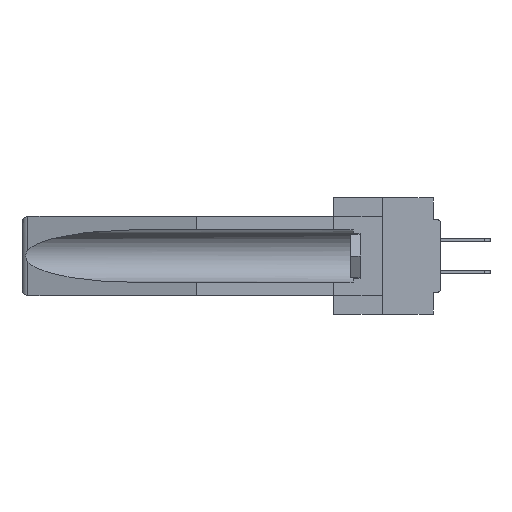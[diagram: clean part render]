
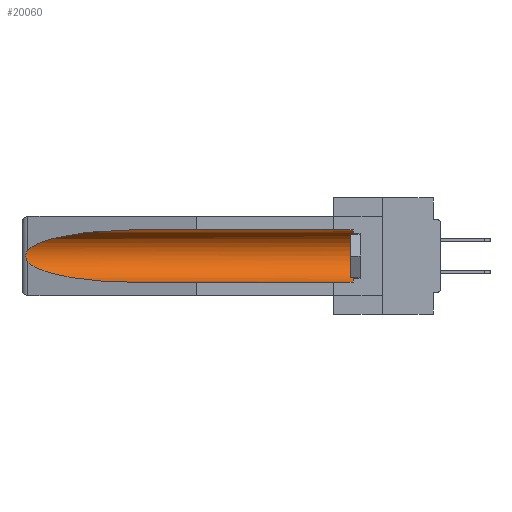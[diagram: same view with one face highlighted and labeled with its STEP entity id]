
A CAD part, left-side view. The second image highlights one B-rep face of the part: STEP entity #20060.
In plain terms, the highlighted cylindrical face has radius 2.857 mm (diameter 5.715 mm), a partial arc.
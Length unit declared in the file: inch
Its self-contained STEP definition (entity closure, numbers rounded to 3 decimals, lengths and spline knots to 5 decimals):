
#20 = CARTESIAN_POINT ( 'NONE',  ( 0.21114, 1.30732, -0.284 ) ) ;
#1206 = CARTESIAN_POINT ( 'NONE',  ( 0.26537, 1.52718, -0.14972 ) ) ;
#1424 = EDGE_CURVE ( 'NONE', #20985, #10053, #11545, .T. ) ;
#1630 = EDGE_CURVE ( 'NONE', #35084, #40783, #12190, .T. ) ;
#1663 = CARTESIAN_POINT ( 'NONE',  ( 0.25451, 1.48313, -0.09465 ) ) ;
#2729 = DIRECTION ( 'NONE',  ( 0., 1., 0. ) ) ;
#2891 = CARTESIAN_POINT ( 'NONE',  ( 0.155, 1.07973, -0.059 ) ) ;
#5031 = DIRECTION ( 'NONE',  ( 0., 1., 0. ) ) ;
#5804 = CARTESIAN_POINT ( 'NONE',  ( 0.2675, 1.53308, -0.16763 ) ) ;
#6280 = VERTEX_POINT ( 'NONE', #25999 ) ;
#8347 = VERTEX_POINT ( 'NONE', #2891 ) ;
#8759 = EDGE_CURVE ( 'NONE', #8347, #35084, #24350, .T. ) ;
#9549 = EDGE_CURVE ( 'NONE', #40783, #10053, #16324, .T. ) ;
#9585 = ORIENTED_EDGE ( 'NONE', *, *, #8759, .T. ) ;
#9876 = CARTESIAN_POINT ( 'NONE',  ( 0.26537, 1.52718, -0.19328 ) ) ;
#10053 = VERTEX_POINT ( 'NONE', #32506 ) ;
#11545 = LINE ( 'NONE', #38792, #32126 ) ;
#12190 = B_SPLINE_CURVE_WITH_KNOTS ( 'NONE', 3,
 ( #27003, #30457, #13221, #40988, #5804, #16128, #20136, #27146, #44496, #23081 ),
 .UNSPECIFIED., .F., .F.,
 ( 4, 2, 2, 2, 4 ),
 ( 0., 0.00029, 0.00058, 0.00087, 0.00117 ),
 .UNSPECIFIED. ) ;
#13221 = CARTESIAN_POINT ( 'NONE',  ( 0.26654, 1.53092, -0.15636 ) ) ;
#13611 = CARTESIAN_POINT ( 'NONE',  ( 0.155, 0.126, -0.1715 ) ) ;
#15307 = CYLINDRICAL_SURFACE ( 'NONE', #31145, 0.1125 ) ;
#16128 = CARTESIAN_POINT ( 'NONE',  ( 0.2675, 1.53308, -0.17534 ) ) ;
#16324 =( BOUNDED_CURVE ( )  B_SPLINE_CURVE ( 3, ( #39674, #37750, #20, #20393 ),
 .UNSPECIFIED., .F., .F. ) 
 B_SPLINE_CURVE_WITH_KNOTS ( ( 4, 4 ),
 ( 0.1948, 1.5708 ),
 .UNSPECIFIED. ) 
 CURVE ( )  GEOMETRIC_REPRESENTATION_ITEM ( )  RATIONAL_B_SPLINE_CURVE ( ( 1., 0.848, 0.848, 1. ) ) 
 REPRESENTATION_ITEM ( '' )  );
#16399 = FACE_OUTER_BOUND ( 'NONE', #27648, .T. ) ;
#16634 = ORIENTED_EDGE ( 'NONE', *, *, #1630, .T. ) ;
#19645 = DIRECTION ( 'NONE',  ( 0., 0., 1. ) ) ;
#20060 = ADVANCED_FACE ( 'NONE', ( #16399 ), #15307, .F. ) ;
#20136 = CARTESIAN_POINT ( 'NONE',  ( 0.2673, 1.53269, -0.17917 ) ) ;
#20393 = CARTESIAN_POINT ( 'NONE',  ( 0.155, 1.07973, -0.284 ) ) ;
#20543 = DIRECTION ( 'NONE',  ( 0., 0., 1. ) ) ;
#20985 = VERTEX_POINT ( 'NONE', #24520 ) ;
#21952 = VECTOR ( 'NONE', #5031, 39.37008 ) ;
#23081 = CARTESIAN_POINT ( 'NONE',  ( 0.26537, 1.52718, -0.19328 ) ) ;
#23207 = ORIENTED_EDGE ( 'NONE', *, *, #23933, .T. ) ;
#23933 = EDGE_CURVE ( 'NONE', #6280, #8347, #32287, .T. ) ;
#24350 =( BOUNDED_CURVE ( )  B_SPLINE_CURVE ( 3, ( #39292, #43068, #1663, #1206 ),
 .UNSPECIFIED., .F., .F. ) 
 B_SPLINE_CURVE_WITH_KNOTS ( ( 4, 4 ),
 ( 4.71239, 6.08839 ),
 .UNSPECIFIED. ) 
 CURVE ( )  GEOMETRIC_REPRESENTATION_ITEM ( )  RATIONAL_B_SPLINE_CURVE ( ( 1., 0.848, 0.848, 1. ) ) 
 REPRESENTATION_ITEM ( '' )  );
#24520 = CARTESIAN_POINT ( 'NONE',  ( 0.155, 0.126, -0.284 ) ) ;
#25999 = CARTESIAN_POINT ( 'NONE',  ( 0.155, 0.126, -0.059 ) ) ;
#27003 = CARTESIAN_POINT ( 'NONE',  ( 0.26537, 1.52718, -0.14972 ) ) ;
#27146 = CARTESIAN_POINT ( 'NONE',  ( 0.26655, 1.53094, -0.18657 ) ) ;
#27648 = EDGE_LOOP ( 'NONE', ( #9585, #16634, #31388, #28370, #41620, #23207 ) ) ;
#28370 = ORIENTED_EDGE ( 'NONE', *, *, #1424, .F. ) ;
#30457 = CARTESIAN_POINT ( 'NONE',  ( 0.26597, 1.52961, -0.15275 ) ) ;
#31145 = AXIS2_PLACEMENT_3D ( 'NONE', #34068, #2729, #19645 ) ;
#31388 = ORIENTED_EDGE ( 'NONE', *, *, #9549, .T. ) ;
#32126 = VECTOR ( 'NONE', #42091, 39.37008 ) ;
#32287 = LINE ( 'NONE', #35805, #21952 ) ;
#32506 = CARTESIAN_POINT ( 'NONE',  ( 0.155, 1.07973, -0.284 ) ) ;
#32802 = CARTESIAN_POINT ( 'NONE',  ( 0.26537, 1.52718, -0.14972 ) ) ;
#34068 = CARTESIAN_POINT ( 'NONE',  ( 0.155, -0.30754, -0.1715 ) ) ;
#35084 = VERTEX_POINT ( 'NONE', #32802 ) ;
#35805 = CARTESIAN_POINT ( 'NONE',  ( 0.155, -0.30754, -0.059 ) ) ;
#37076 = CIRCLE ( 'NONE', #39961, 0.1125 ) ;
#37750 = CARTESIAN_POINT ( 'NONE',  ( 0.25451, 1.48313, -0.24835 ) ) ;
#38792 = CARTESIAN_POINT ( 'NONE',  ( 0.155, -0.30754, -0.284 ) ) ;
#39292 = CARTESIAN_POINT ( 'NONE',  ( 0.155, 1.07973, -0.059 ) ) ;
#39674 = CARTESIAN_POINT ( 'NONE',  ( 0.26537, 1.52718, -0.19328 ) ) ;
#39961 = AXIS2_PLACEMENT_3D ( 'NONE', #13611, #41385, #20543 ) ;
#40783 = VERTEX_POINT ( 'NONE', #9876 ) ;
#40988 = CARTESIAN_POINT ( 'NONE',  ( 0.2673, 1.5327, -0.16383 ) ) ;
#41173 = EDGE_CURVE ( 'NONE', #20985, #6280, #37076, .T. ) ;
#41385 = DIRECTION ( 'NONE',  ( 0., -1., 0. ) ) ;
#41620 = ORIENTED_EDGE ( 'NONE', *, *, #41173, .T. ) ;
#42091 = DIRECTION ( 'NONE',  ( 0., 1., 0. ) ) ;
#43068 = CARTESIAN_POINT ( 'NONE',  ( 0.21114, 1.30732, -0.059 ) ) ;
#44496 = CARTESIAN_POINT ( 'NONE',  ( 0.26597, 1.5296, -0.19026 ) ) ;
